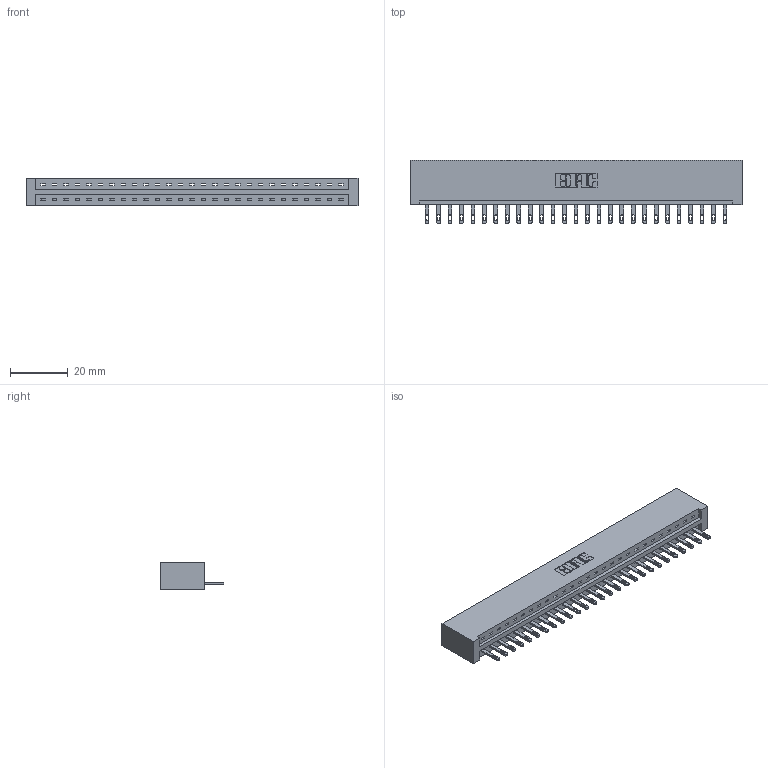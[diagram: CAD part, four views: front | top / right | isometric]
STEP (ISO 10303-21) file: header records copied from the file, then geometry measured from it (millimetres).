
FILE_DESCRIPTION (( 'STEP AP203' ), '1' );
FILE_NAME ('887-027-500-101.STEP', '2020-09-20T19:46:58', ( '' ), ( '' ), 'SwSTEP 2.0', 'SolidWorks 2020', '' );
FILE_SCHEMA (( 'CONFIG_CONTROL_DESIGN' ));
Length unit declared in the file: inch
Products named in the file (3): 345-292-001_345-293-100; 837 Part_No Mounting Lugs; 887-027-500-101
Assembly tree (28 placements, depth 2):
  887-027-500-101
    837 Part_No Mounting Lugs
    345-292-001_345-293-100  x27
Bounding box: 114.86 x 21.85 x 9.4 mm (x, y, z)
Volume: 12505.4 mm3; surface area: 12883.7 mm2
Topology: 28 solids, 28 shells, 1672 faces, 5147 edges, 3430 vertices
Faces by surface type: plane 1146, cylinder 526
Entity records: 21663 total; most frequent: CARTESIAN_POINT 3779, ORIENTED_EDGE 3742, DIRECTION 3205, EDGE_CURVE 1871, VECTOR 1747, LINE 1747, VERTEX_POINT 1246, AXIS2_PLACEMENT_3D 729
